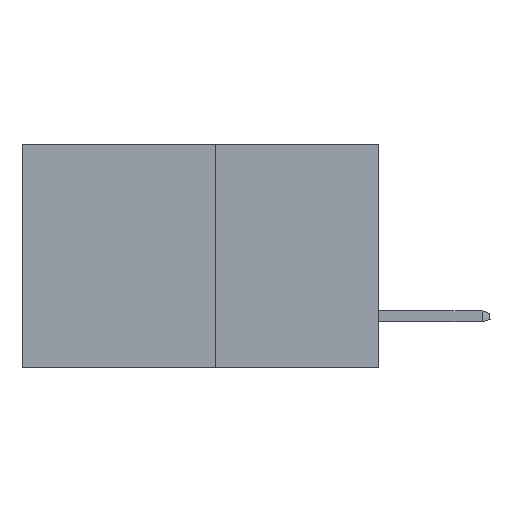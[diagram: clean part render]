
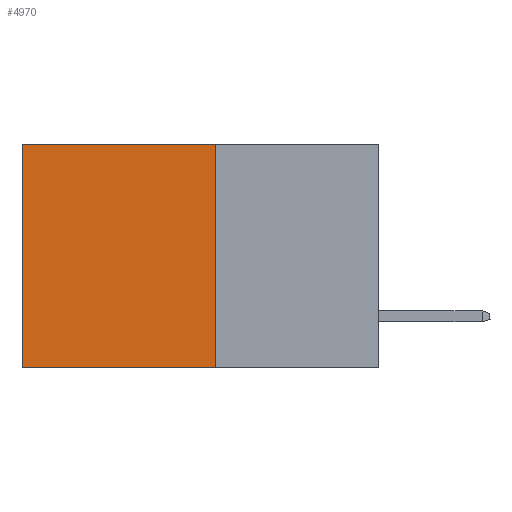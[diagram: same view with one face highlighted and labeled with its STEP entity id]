
A CAD part, left-side view. The second image highlights one B-rep face of the part: STEP entity #4970.
In plain terms, the highlighted planar face has unit normal (-1, 0, 0).
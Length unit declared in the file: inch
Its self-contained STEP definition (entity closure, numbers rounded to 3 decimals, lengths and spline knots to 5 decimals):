
#197 = ORIENTED_EDGE ( 'NONE', *, *, #15298, .F. ) ;
#584 = CARTESIAN_POINT ( 'NONE',  ( 0.277, 0.27, 0. ) ) ;
#1171 = CARTESIAN_POINT ( 'NONE',  ( 0.277, 0.59, 0. ) ) ;
#1183 = CARTESIAN_POINT ( 'NONE',  ( 0.277, 0.27, 0. ) ) ;
#1647 = DIRECTION ( 'NONE',  ( 0., 0., -1. ) ) ;
#1714 = DIRECTION ( 'NONE',  ( 1., 0., 0. ) ) ;
#2278 = ORIENTED_EDGE ( 'NONE', *, *, #6389, .T. ) ;
#2682 = EDGE_CURVE ( 'NONE', #17841, #9189, #10403, .T. ) ;
#2694 = ORIENTED_EDGE ( 'NONE', *, *, #2682, .F. ) ;
#3106 = ORIENTED_EDGE ( 'NONE', *, *, #13033, .T. ) ;
#3490 = LINE ( 'NONE', #1183, #19237 ) ;
#3552 = VERTEX_POINT ( 'NONE', #1171 ) ;
#3869 = EDGE_LOOP ( 'NONE', ( #2278, #2694, #197, #3106 ) ) ;
#4380 = DIRECTION ( 'NONE',  ( 0., 1., 0. ) ) ;
#4970 = ADVANCED_FACE ( 'NONE', ( #12873 ), #13158, .F. ) ;
#5679 = VECTOR ( 'NONE', #19573, 39.37008 ) ;
#6389 = EDGE_CURVE ( 'NONE', #3552, #9189, #17335, .T. ) ;
#6401 = DIRECTION ( 'NONE',  ( 0., 0., -1. ) ) ;
#9189 = VERTEX_POINT ( 'NONE', #11767 ) ;
#10403 = LINE ( 'NONE', #10481, #18365 ) ;
#10481 = CARTESIAN_POINT ( 'NONE',  ( 0.277, 0.27, -0.37 ) ) ;
#10561 = DIRECTION ( 'NONE',  ( 0., 1., 0. ) ) ;
#10970 = CARTESIAN_POINT ( 'NONE',  ( 0.277, 0.27, -0.37 ) ) ;
#11767 = CARTESIAN_POINT ( 'NONE',  ( 0.277, 0.59, -0.37 ) ) ;
#11907 = LINE ( 'NONE', #10970, #15486 ) ;
#12873 = FACE_OUTER_BOUND ( 'NONE', #3869, .T. ) ;
#13033 = EDGE_CURVE ( 'NONE', #18668, #3552, #3490, .T. ) ;
#13158 = PLANE ( 'NONE',  #14889 ) ;
#13428 = CARTESIAN_POINT ( 'NONE',  ( 0.277, 0.27, -0.37 ) ) ;
#14889 = AXIS2_PLACEMENT_3D ( 'NONE', #13428, #1714, #1647 ) ;
#15298 = EDGE_CURVE ( 'NONE', #18668, #17841, #11907, .T. ) ;
#15486 = VECTOR ( 'NONE', #6401, 39.37008 ) ;
#15595 = CARTESIAN_POINT ( 'NONE',  ( 0.277, 0.27, -0.37 ) ) ;
#17335 = LINE ( 'NONE', #18242, #5679 ) ;
#17841 = VERTEX_POINT ( 'NONE', #15595 ) ;
#18242 = CARTESIAN_POINT ( 'NONE',  ( 0.277, 0.59, -0.37 ) ) ;
#18365 = VECTOR ( 'NONE', #10561, 39.37008 ) ;
#18668 = VERTEX_POINT ( 'NONE', #584 ) ;
#19237 = VECTOR ( 'NONE', #4380, 39.37008 ) ;
#19573 = DIRECTION ( 'NONE',  ( 0., 0., -1. ) ) ;
